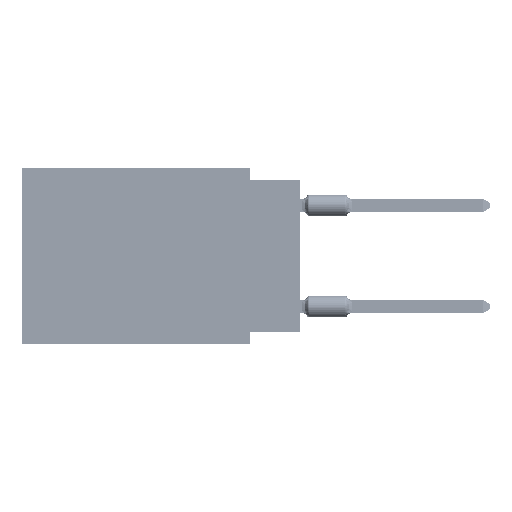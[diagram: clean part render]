
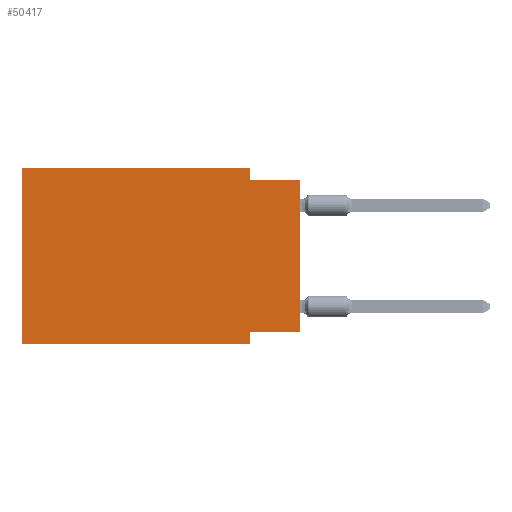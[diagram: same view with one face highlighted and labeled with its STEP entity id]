
A CAD part, left-side view. The second image highlights one B-rep face of the part: STEP entity #50417.
In plain terms, the highlighted planar face has unit normal (-1, 0, 0).
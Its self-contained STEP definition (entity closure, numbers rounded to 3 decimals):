
#3230 = LINE ( 'NONE', #75554, #20904 ) ;
#9219 = VERTEX_POINT ( 'NONE', #68318 ) ;
#9324 = LINE ( 'NONE', #61118, #80759 ) ;
#10653 = VERTEX_POINT ( 'NONE', #48580 ) ;
#11158 = EDGE_CURVE ( 'NONE', #30627, #72155, #75469, .T. ) ;
#13185 = VERTEX_POINT ( 'NONE', #29486 ) ;
#13635 = EDGE_CURVE ( 'NONE', #68798, #36121, #80753, .T. ) ;
#14485 = ORIENTED_EDGE ( 'NONE', *, *, #48454, .F. ) ;
#14771 = VERTEX_POINT ( 'NONE', #49326 ) ;
#18612 = EDGE_CURVE ( 'NONE', #10653, #9219, #3230, .T. ) ;
#20904 = VECTOR ( 'NONE', #48565, 1000. ) ;
#27368 = VECTOR ( 'NONE', #35546, 1000. ) ;
#28521 = DIRECTION ( 'NONE',  ( 0., -1., 0. ) ) ;
#29000 = DIRECTION ( 'NONE',  ( 0., -1., 0. ) ) ;
#29486 = CARTESIAN_POINT ( 'NONE',  ( 0., 13.97, 0. ) ) ;
#29930 = VECTOR ( 'NONE', #29000, 1000. ) ;
#30096 = VECTOR ( 'NONE', #28521, 1000. ) ;
#30627 = VERTEX_POINT ( 'NONE', #62374 ) ;
#31509 = CARTESIAN_POINT ( 'NONE',  ( 0., 13.97, 0. ) ) ;
#32678 = ORIENTED_EDGE ( 'NONE', *, *, #38322, .F. ) ;
#33098 = LINE ( 'NONE', #48371, #27368 ) ;
#33429 = ORIENTED_EDGE ( 'NONE', *, *, #42105, .F. ) ;
#34360 = CARTESIAN_POINT ( 'NONE',  ( 0., 0., -8.255 ) ) ;
#35546 = DIRECTION ( 'NONE',  ( 0., 0., -1. ) ) ;
#36121 = VERTEX_POINT ( 'NONE', #51497 ) ;
#37836 = CARTESIAN_POINT ( 'NONE',  ( 0., 0., -0.635 ) ) ;
#38322 = EDGE_CURVE ( 'NONE', #68798, #13185, #9324, .T. ) ;
#38782 = DIRECTION ( 'NONE',  ( 1., 0., 0. ) ) ;
#40950 = CARTESIAN_POINT ( 'NONE',  ( 0., 13.97, -8.89 ) ) ;
#41824 = LINE ( 'NONE', #37836, #29930 ) ;
#42105 = EDGE_CURVE ( 'NONE', #13185, #10653, #46729, .T. ) ;
#44506 = ORIENTED_EDGE ( 'NONE', *, *, #18612, .F. ) ;
#45625 = CARTESIAN_POINT ( 'NONE',  ( 0., 0., -0.635 ) ) ;
#46507 = EDGE_CURVE ( 'NONE', #9219, #72155, #41824, .T. ) ;
#46717 = EDGE_CURVE ( 'NONE', #30627, #14771, #54038, .T. ) ;
#46729 = LINE ( 'NONE', #68101, #59412 ) ;
#46883 = ORIENTED_EDGE ( 'NONE', *, *, #46507, .F. ) ;
#48371 = CARTESIAN_POINT ( 'NONE',  ( 0., 2.54, -8.89 ) ) ;
#48454 = EDGE_CURVE ( 'NONE', #14771, #36121, #33098, .T. ) ;
#48565 = DIRECTION ( 'NONE',  ( 0., 0., -1. ) ) ;
#48580 = CARTESIAN_POINT ( 'NONE',  ( 0., 2.54, 0. ) ) ;
#49326 = CARTESIAN_POINT ( 'NONE',  ( 0., 2.54, -8.255 ) ) ;
#50417 = ADVANCED_FACE ( 'NONE', ( #82904 ), #56787, .F. ) ;
#51497 = CARTESIAN_POINT ( 'NONE',  ( 0., 2.54, -8.89 ) ) ;
#54038 = LINE ( 'NONE', #34360, #57229 ) ;
#54071 = CARTESIAN_POINT ( 'NONE',  ( 0., 0., 0. ) ) ;
#54370 = ORIENTED_EDGE ( 'NONE', *, *, #13635, .T. ) ;
#54408 = DIRECTION ( 'NONE',  ( 0., -1., 0. ) ) ;
#55115 = DIRECTION ( 'NONE',  ( 0., 0., 1. ) ) ;
#56787 = PLANE ( 'NONE',  #82055 ) ;
#57229 = VECTOR ( 'NONE', #80162, 1000. ) ;
#59391 = VECTOR ( 'NONE', #80193, 1000. ) ;
#59412 = VECTOR ( 'NONE', #54408, 1000. ) ;
#61118 = CARTESIAN_POINT ( 'NONE',  ( 0., 13.97, 0. ) ) ;
#62027 = EDGE_LOOP ( 'NONE', ( #84571, #46883, #44506, #33429, #32678, #54370, #14485, #84104 ) ) ;
#62374 = CARTESIAN_POINT ( 'NONE',  ( 0., 0., -8.255 ) ) ;
#68101 = CARTESIAN_POINT ( 'NONE',  ( 0., 13.97, 0. ) ) ;
#68318 = CARTESIAN_POINT ( 'NONE',  ( 0., 2.54, -0.635 ) ) ;
#68798 = VERTEX_POINT ( 'NONE', #70734 ) ;
#70734 = CARTESIAN_POINT ( 'NONE',  ( 0., 13.97, -8.89 ) ) ;
#72155 = VERTEX_POINT ( 'NONE', #45625 ) ;
#75469 = LINE ( 'NONE', #54071, #59391 ) ;
#75554 = CARTESIAN_POINT ( 'NONE',  ( 0., 2.54, 0. ) ) ;
#76905 = DIRECTION ( 'NONE',  ( 0., 0., -1. ) ) ;
#80162 = DIRECTION ( 'NONE',  ( 0., 1., 0. ) ) ;
#80193 = DIRECTION ( 'NONE',  ( 0., 0., 1. ) ) ;
#80753 = LINE ( 'NONE', #40950, #30096 ) ;
#80759 = VECTOR ( 'NONE', #55115, 1000. ) ;
#82055 = AXIS2_PLACEMENT_3D ( 'NONE', #31509, #38782, #76905 ) ;
#82904 = FACE_OUTER_BOUND ( 'NONE', #62027, .T. ) ;
#84104 = ORIENTED_EDGE ( 'NONE', *, *, #46717, .F. ) ;
#84571 = ORIENTED_EDGE ( 'NONE', *, *, #11158, .T. ) ;
